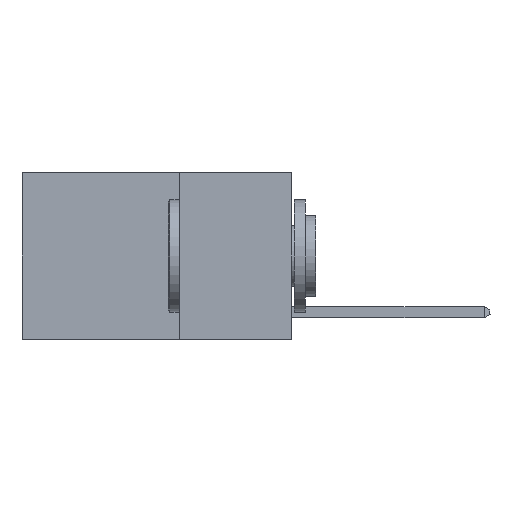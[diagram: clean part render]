
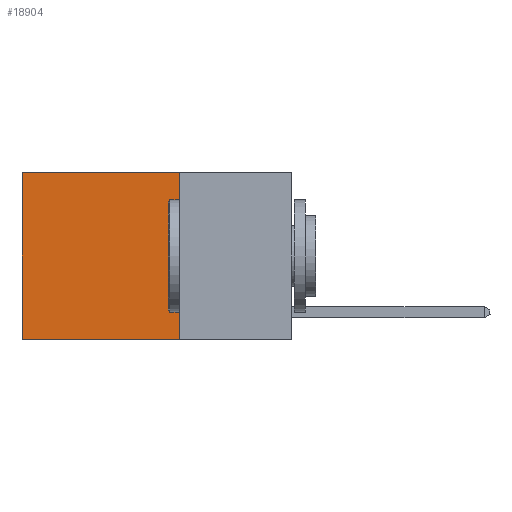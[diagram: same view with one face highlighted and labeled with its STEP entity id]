
A CAD part, left-side view. The second image highlights one B-rep face of the part: STEP entity #18904.
In plain terms, the highlighted planar face has unit normal (-1, 0, 0).
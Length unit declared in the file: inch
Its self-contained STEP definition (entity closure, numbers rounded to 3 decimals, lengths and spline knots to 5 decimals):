
#1487 = DIRECTION ( 'NONE',  ( 0., 0., -1. ) ) ;
#2022 = DIRECTION ( 'NONE',  ( 0., 1., 0. ) ) ;
#2561 = CARTESIAN_POINT ( 'NONE',  ( 0.2625, 0.25, -0.37 ) ) ;
#3078 = CARTESIAN_POINT ( 'NONE',  ( 0.2625, 0.25, -0.37 ) ) ;
#3920 = LINE ( 'NONE', #22696, #13789 ) ;
#4602 = DIRECTION ( 'NONE',  ( 1., 0., 0. ) ) ;
#5166 = VERTEX_POINT ( 'NONE', #3078 ) ;
#5200 = VECTOR ( 'NONE', #2022, 39.37008 ) ;
#5521 = LINE ( 'NONE', #27078, #8345 ) ;
#7119 = AXIS2_PLACEMENT_3D ( 'NONE', #13266, #4602, #23784 ) ;
#8326 = ORIENTED_EDGE ( 'NONE', *, *, #8924, .F. ) ;
#8345 = VECTOR ( 'NONE', #1487, 39.37008 ) ;
#8924 = EDGE_CURVE ( 'NONE', #5166, #19026, #15303, .T. ) ;
#9036 = CARTESIAN_POINT ( 'NONE',  ( 0.2625, 0.6, 0. ) ) ;
#9341 = CARTESIAN_POINT ( 'NONE',  ( 0.2625, 0.6, -0.37 ) ) ;
#10895 = FACE_OUTER_BOUND ( 'NONE', #17324, .T. ) ;
#11032 = ORIENTED_EDGE ( 'NONE', *, *, #15290, .F. ) ;
#11641 = ORIENTED_EDGE ( 'NONE', *, *, #26895, .T. ) ;
#11955 = ORIENTED_EDGE ( 'NONE', *, *, #14094, .T. ) ;
#12636 = CARTESIAN_POINT ( 'NONE',  ( 0.2625, 0.25, 0. ) ) ;
#13266 = CARTESIAN_POINT ( 'NONE',  ( 0.2625, 0.25, 0. ) ) ;
#13789 = VECTOR ( 'NONE', #18481, 39.37008 ) ;
#14094 = EDGE_CURVE ( 'NONE', #15459, #23426, #25384, .T. ) ;
#15243 = PLANE ( 'NONE',  #7119 ) ;
#15290 = EDGE_CURVE ( 'NONE', #15459, #5166, #5521, .T. ) ;
#15303 = LINE ( 'NONE', #2561, #20183 ) ;
#15459 = VERTEX_POINT ( 'NONE', #16986 ) ;
#16986 = CARTESIAN_POINT ( 'NONE',  ( 0.2625, 0.25, 0. ) ) ;
#17324 = EDGE_LOOP ( 'NONE', ( #11641, #8326, #11032, #11955 ) ) ;
#18481 = DIRECTION ( 'NONE',  ( 0., 0., -1. ) ) ;
#18904 = ADVANCED_FACE ( 'NONE', ( #10895 ), #15243, .F. ) ;
#19026 = VERTEX_POINT ( 'NONE', #9341 ) ;
#20183 = VECTOR ( 'NONE', #24127, 39.37008 ) ;
#22696 = CARTESIAN_POINT ( 'NONE',  ( 0.2625, 0.6, 0. ) ) ;
#23426 = VERTEX_POINT ( 'NONE', #9036 ) ;
#23784 = DIRECTION ( 'NONE',  ( 0., 0., -1. ) ) ;
#24127 = DIRECTION ( 'NONE',  ( 0., 1., 0. ) ) ;
#25384 = LINE ( 'NONE', #12636, #5200 ) ;
#26895 = EDGE_CURVE ( 'NONE', #23426, #19026, #3920, .T. ) ;
#27078 = CARTESIAN_POINT ( 'NONE',  ( 0.2625, 0.25, 0. ) ) ;
